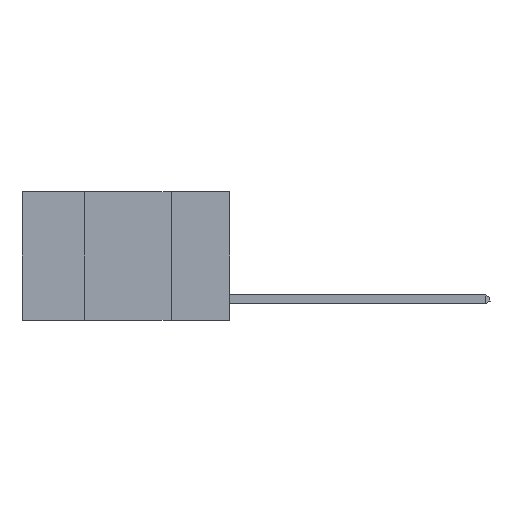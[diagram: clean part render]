
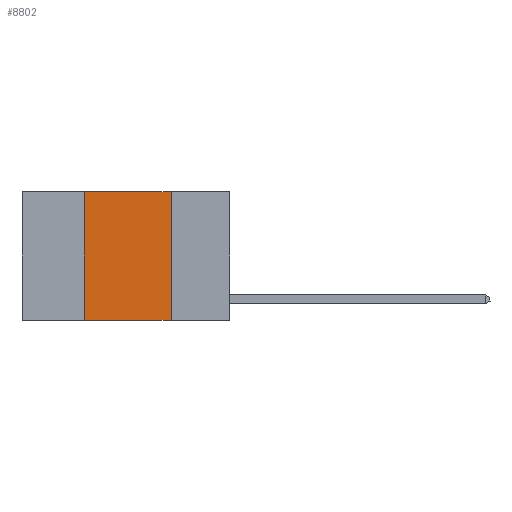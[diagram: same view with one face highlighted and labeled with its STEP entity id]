
A CAD part, left-side view. The second image highlights one B-rep face of the part: STEP entity #8802.
In plain terms, the highlighted planar face has unit normal (-1, 0, 0).
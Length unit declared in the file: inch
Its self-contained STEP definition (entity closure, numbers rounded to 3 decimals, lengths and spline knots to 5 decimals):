
#151 = FACE_OUTER_BOUND ( 'NONE', #5344, .T. ) ;
#674 = EDGE_CURVE ( 'NONE', #8473, #10333, #12851, .T. ) ;
#1053 = LINE ( 'NONE', #5166, #1579 ) ;
#1482 = VECTOR ( 'NONE', #9913, 39.37008 ) ;
#1579 = VECTOR ( 'NONE', #11009, 39.37008 ) ;
#2394 = DIRECTION ( 'NONE',  ( 1., 0., 0. ) ) ;
#2502 = DIRECTION ( 'NONE',  ( 0., -1., 0. ) ) ;
#2784 = CARTESIAN_POINT ( 'NONE',  ( 0., 0.17, 0. ) ) ;
#3230 = CARTESIAN_POINT ( 'NONE',  ( 0., 0.42, -0.37 ) ) ;
#3290 = EDGE_CURVE ( 'NONE', #5207, #8884, #8568, .T. ) ;
#3405 = CARTESIAN_POINT ( 'NONE',  ( 0., 0.6, 0. ) ) ;
#4024 = EDGE_CURVE ( 'NONE', #8473, #5207, #1053, .T. ) ;
#4192 = ORIENTED_EDGE ( 'NONE', *, *, #11805, .F. ) ;
#5166 = CARTESIAN_POINT ( 'NONE',  ( 0., 0.42, 0. ) ) ;
#5207 = VERTEX_POINT ( 'NONE', #8563 ) ;
#5313 = DIRECTION ( 'NONE',  ( 0., 0., -1. ) ) ;
#5344 = EDGE_LOOP ( 'NONE', ( #4192, #7569, #9946, #6810 ) ) ;
#5427 = CARTESIAN_POINT ( 'NONE',  ( 0., 0.17, 0. ) ) ;
#5465 = CARTESIAN_POINT ( 'NONE',  ( 0., 0.17, -0.37 ) ) ;
#6270 = VECTOR ( 'NONE', #2502, 39.37008 ) ;
#6810 = ORIENTED_EDGE ( 'NONE', *, *, #674, .T. ) ;
#7273 = AXIS2_PLACEMENT_3D ( 'NONE', #3405, #2394, #5313 ) ;
#7569 = ORIENTED_EDGE ( 'NONE', *, *, #3290, .F. ) ;
#7645 = VECTOR ( 'NONE', #11087, 39.37008 ) ;
#8451 = PLANE ( 'NONE',  #7273 ) ;
#8473 = VERTEX_POINT ( 'NONE', #3230 ) ;
#8563 = CARTESIAN_POINT ( 'NONE',  ( 0., 0.42, 0. ) ) ;
#8568 = LINE ( 'NONE', #12725, #6270 ) ;
#8802 = ADVANCED_FACE ( 'NONE', ( #151 ), #8451, .F. ) ;
#8884 = VERTEX_POINT ( 'NONE', #5427 ) ;
#9913 = DIRECTION ( 'NONE',  ( 0., -1., 0. ) ) ;
#9946 = ORIENTED_EDGE ( 'NONE', *, *, #4024, .F. ) ;
#10333 = VERTEX_POINT ( 'NONE', #5465 ) ;
#10926 = CARTESIAN_POINT ( 'NONE',  ( 0., 0.6, -0.37 ) ) ;
#11009 = DIRECTION ( 'NONE',  ( 0., 0., 1. ) ) ;
#11087 = DIRECTION ( 'NONE',  ( 0., 0., -1. ) ) ;
#11805 = EDGE_CURVE ( 'NONE', #8884, #10333, #13136, .T. ) ;
#12725 = CARTESIAN_POINT ( 'NONE',  ( 0., 0.6, 0. ) ) ;
#12851 = LINE ( 'NONE', #10926, #1482 ) ;
#13136 = LINE ( 'NONE', #2784, #7645 ) ;
